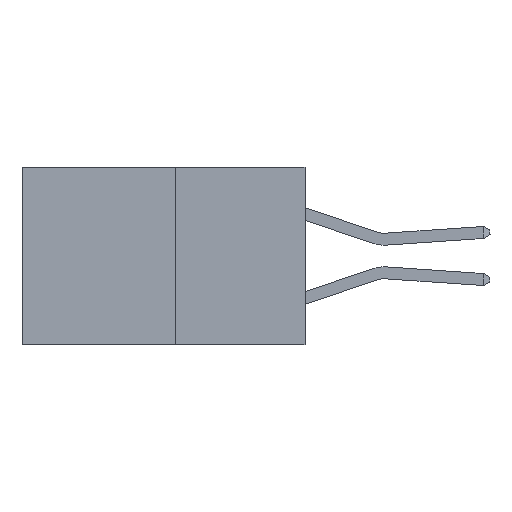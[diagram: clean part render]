
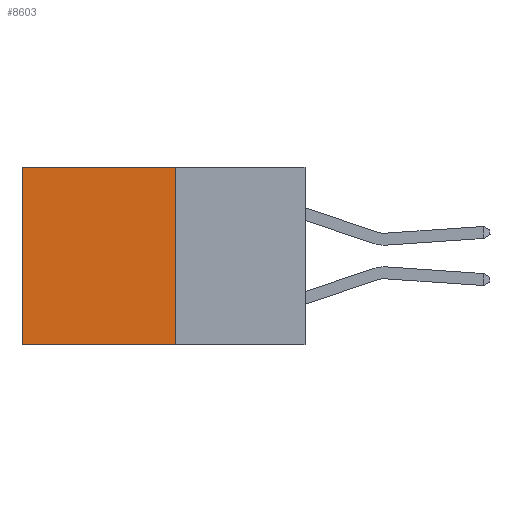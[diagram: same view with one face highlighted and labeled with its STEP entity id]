
A CAD part, left-side view. The second image highlights one B-rep face of the part: STEP entity #8603.
In plain terms, the highlighted planar face has unit normal (-1, 0, 0).
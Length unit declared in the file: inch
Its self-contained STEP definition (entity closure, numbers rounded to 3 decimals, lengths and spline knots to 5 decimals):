
#599 = CARTESIAN_POINT ( 'NONE',  ( 0.277, 0.27, -0.37 ) ) ;
#1819 = CARTESIAN_POINT ( 'NONE',  ( 0.277, 0.59, -0.37 ) ) ;
#1849 = LINE ( 'NONE', #8654, #11809 ) ;
#1937 = VERTEX_POINT ( 'NONE', #9322 ) ;
#2814 = ORIENTED_EDGE ( 'NONE', *, *, #15673, .T. ) ;
#3917 = LINE ( 'NONE', #6115, #13736 ) ;
#3943 = CARTESIAN_POINT ( 'NONE',  ( 0.277, 0.59, 0. ) ) ;
#4285 = VERTEX_POINT ( 'NONE', #5074 ) ;
#5074 = CARTESIAN_POINT ( 'NONE',  ( 0.277, 0.27, -0.37 ) ) ;
#5274 = VERTEX_POINT ( 'NONE', #1819 ) ;
#6023 = ORIENTED_EDGE ( 'NONE', *, *, #8995, .T. ) ;
#6115 = CARTESIAN_POINT ( 'NONE',  ( 0.277, 0.27, -0.37 ) ) ;
#7108 = DIRECTION ( 'NONE',  ( 1., 0., 0. ) ) ;
#8364 = FACE_OUTER_BOUND ( 'NONE', #9428, .T. ) ;
#8603 = ADVANCED_FACE ( 'NONE', ( #8364 ), #9959, .F. ) ;
#8654 = CARTESIAN_POINT ( 'NONE',  ( 0.277, 0.27, 0. ) ) ;
#8728 = CARTESIAN_POINT ( 'NONE',  ( 0.277, 0.59, -0.37 ) ) ;
#8995 = EDGE_CURVE ( 'NONE', #10656, #5274, #16283, .T. ) ;
#9128 = VECTOR ( 'NONE', #13509, 39.37008 ) ;
#9322 = CARTESIAN_POINT ( 'NONE',  ( 0.277, 0.27, 0. ) ) ;
#9428 = EDGE_LOOP ( 'NONE', ( #6023, #15759, #13717, #2814 ) ) ;
#9882 = CARTESIAN_POINT ( 'NONE',  ( 0.277, 0.27, -0.37 ) ) ;
#9919 = DIRECTION ( 'NONE',  ( 0., 1., 0. ) ) ;
#9938 = DIRECTION ( 'NONE',  ( 0., 0., -1. ) ) ;
#9959 = PLANE ( 'NONE',  #12348 ) ;
#10656 = VERTEX_POINT ( 'NONE', #3943 ) ;
#11062 = DIRECTION ( 'NONE',  ( 0., 1., 0. ) ) ;
#11077 = EDGE_CURVE ( 'NONE', #1937, #4285, #3917, .T. ) ;
#11809 = VECTOR ( 'NONE', #9919, 39.37008 ) ;
#12348 = AXIS2_PLACEMENT_3D ( 'NONE', #9882, #7108, #13483 ) ;
#13228 = LINE ( 'NONE', #599, #16185 ) ;
#13483 = DIRECTION ( 'NONE',  ( 0., 0., -1. ) ) ;
#13509 = DIRECTION ( 'NONE',  ( 0., 0., -1. ) ) ;
#13717 = ORIENTED_EDGE ( 'NONE', *, *, #11077, .F. ) ;
#13736 = VECTOR ( 'NONE', #9938, 39.37008 ) ;
#14927 = EDGE_CURVE ( 'NONE', #4285, #5274, #13228, .T. ) ;
#15673 = EDGE_CURVE ( 'NONE', #1937, #10656, #1849, .T. ) ;
#15759 = ORIENTED_EDGE ( 'NONE', *, *, #14927, .F. ) ;
#16185 = VECTOR ( 'NONE', #11062, 39.37008 ) ;
#16283 = LINE ( 'NONE', #8728, #9128 ) ;
